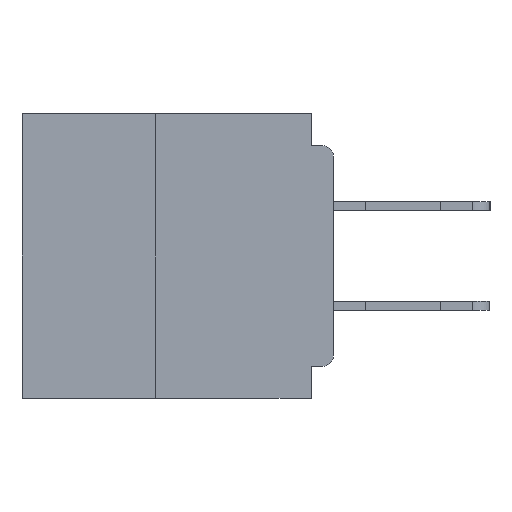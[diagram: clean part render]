
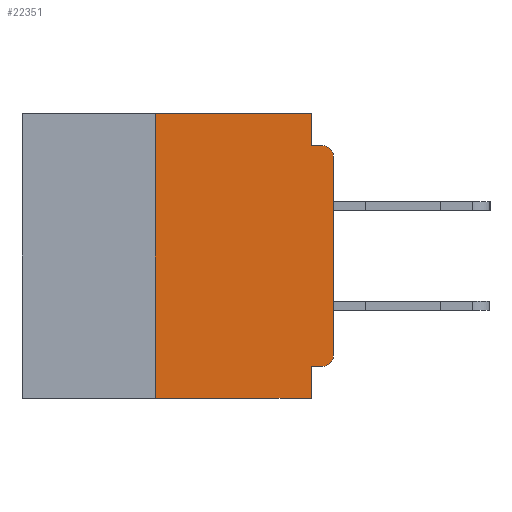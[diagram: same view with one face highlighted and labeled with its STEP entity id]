
A CAD part, left-side view. The second image highlights one B-rep face of the part: STEP entity #22351.
In plain terms, the highlighted planar face has unit normal (-1, 0, 0).
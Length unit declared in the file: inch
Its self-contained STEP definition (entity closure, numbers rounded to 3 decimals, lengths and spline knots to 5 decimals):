
#39 = VERTEX_POINT ( 'NONE', #34065 ) ;
#1166 = EDGE_CURVE ( 'NONE', #16202, #13693, #30285, .T. ) ;
#1702 = CARTESIAN_POINT ( 'NONE',  ( 0., 0., -0.045 ) ) ;
#1745 = EDGE_CURVE ( 'NONE', #2327, #4571, #15936, .T. ) ;
#2327 = VERTEX_POINT ( 'NONE', #35479 ) ;
#2402 = ORIENTED_EDGE ( 'NONE', *, *, #14206, .F. ) ;
#2523 = ORIENTED_EDGE ( 'NONE', *, *, #1745, .T. ) ;
#3564 = CARTESIAN_POINT ( 'NONE',  ( 0., 0.031, -0.4 ) ) ;
#4571 = VERTEX_POINT ( 'NONE', #23631 ) ;
#5161 = DIRECTION ( 'NONE',  ( 1., 0., 0. ) ) ;
#5773 = VERTEX_POINT ( 'NONE', #30542 ) ;
#6461 = ORIENTED_EDGE ( 'NONE', *, *, #18752, .T. ) ;
#7324 = VECTOR ( 'NONE', #26563, 39.37008 ) ;
#7698 = VECTOR ( 'NONE', #8587, 39.37008 ) ;
#8587 = DIRECTION ( 'NONE',  ( 0., 0., 1. ) ) ;
#9088 = EDGE_CURVE ( 'NONE', #33214, #16202, #17918, .T. ) ;
#9130 = LINE ( 'NONE', #1702, #14126 ) ;
#9551 = CARTESIAN_POINT ( 'NONE',  ( 0., 0.031, 0. ) ) ;
#10005 = CARTESIAN_POINT ( 'NONE',  ( 0., 0., -0.355 ) ) ;
#10224 = VECTOR ( 'NONE', #25050, 39.37008 ) ;
#10662 = DIRECTION ( 'NONE',  ( 0., -1., 0. ) ) ;
#10870 = CARTESIAN_POINT ( 'NONE',  ( 0., 0.031, 0. ) ) ;
#10946 = PLANE ( 'NONE',  #32165 ) ;
#11041 = LINE ( 'NONE', #35198, #7324 ) ;
#11042 = CARTESIAN_POINT ( 'NONE',  ( 0., 0.015, -0.34 ) ) ;
#11160 = CARTESIAN_POINT ( 'NONE',  ( 0., 0.031, -0.045 ) ) ;
#13007 = ORIENTED_EDGE ( 'NONE', *, *, #33110, .F. ) ;
#13212 = LINE ( 'NONE', #27355, #27936 ) ;
#13385 = ORIENTED_EDGE ( 'NONE', *, *, #31319, .F. ) ;
#13693 = VERTEX_POINT ( 'NONE', #11160 ) ;
#13855 = CARTESIAN_POINT ( 'NONE',  ( 0., 0.437, 0. ) ) ;
#13951 = DIRECTION ( 'NONE',  ( 0., 0., -1. ) ) ;
#14126 = VECTOR ( 'NONE', #10662, 39.37008 ) ;
#14144 = VERTEX_POINT ( 'NONE', #16159 ) ;
#14206 = EDGE_CURVE ( 'NONE', #5773, #27814, #21734, .T. ) ;
#15553 = VERTEX_POINT ( 'NONE', #28361 ) ;
#15936 = CIRCLE ( 'NONE', #16448, 0.015 ) ;
#16159 = CARTESIAN_POINT ( 'NONE',  ( 0., 0.015, -0.355 ) ) ;
#16202 = VERTEX_POINT ( 'NONE', #10870 ) ;
#16414 = CARTESIAN_POINT ( 'NONE',  ( 0., 0.031, -0.4 ) ) ;
#16448 = AXIS2_PLACEMENT_3D ( 'NONE', #22182, #21031, #35310 ) ;
#17918 = LINE ( 'NONE', #27908, #10224 ) ;
#18578 = EDGE_CURVE ( 'NONE', #13693, #4571, #9130, .T. ) ;
#18752 = EDGE_CURVE ( 'NONE', #15553, #2327, #23318, .T. ) ;
#20002 = VECTOR ( 'NONE', #33392, 39.37008 ) ;
#20537 = VECTOR ( 'NONE', #23725, 39.37008 ) ;
#21031 = DIRECTION ( 'NONE',  ( -1., 0., 0. ) ) ;
#21053 = FACE_OUTER_BOUND ( 'NONE', #37218, .T. ) ;
#21326 = AXIS2_PLACEMENT_3D ( 'NONE', #11042, #31537, #13951 ) ;
#21472 = ORIENTED_EDGE ( 'NONE', *, *, #9088, .F. ) ;
#21734 = LINE ( 'NONE', #16414, #27782 ) ;
#22182 = CARTESIAN_POINT ( 'NONE',  ( 0., 0.015, -0.06 ) ) ;
#22351 = ADVANCED_FACE ( 'NONE', ( #21053 ), #10946, .F. ) ;
#22918 = EDGE_CURVE ( 'NONE', #14144, #15553, #24308, .T. ) ;
#23318 = LINE ( 'NONE', #26151, #7698 ) ;
#23631 = CARTESIAN_POINT ( 'NONE',  ( 0., 0.015, -0.045 ) ) ;
#23725 = DIRECTION ( 'NONE',  ( 0., 0., -1. ) ) ;
#24308 = CIRCLE ( 'NONE', #21326, 0.015 ) ;
#24393 = DIRECTION ( 'NONE',  ( 0., -1., 0. ) ) ;
#24507 = ORIENTED_EDGE ( 'NONE', *, *, #22918, .T. ) ;
#24801 = ORIENTED_EDGE ( 'NONE', *, *, #18578, .F. ) ;
#25050 = DIRECTION ( 'NONE',  ( 0., -1., 0. ) ) ;
#25674 = DIRECTION ( 'NONE',  ( 0., 0., -1. ) ) ;
#25874 = ORIENTED_EDGE ( 'NONE', *, *, #26715, .T. ) ;
#26151 = CARTESIAN_POINT ( 'NONE',  ( 0., 0., 0. ) ) ;
#26563 = DIRECTION ( 'NONE',  ( 0., 0., 1. ) ) ;
#26715 = EDGE_CURVE ( 'NONE', #39, #27814, #13212, .T. ) ;
#27355 = CARTESIAN_POINT ( 'NONE',  ( 0., 0.437, -0.4 ) ) ;
#27782 = VECTOR ( 'NONE', #33985, 39.37008 ) ;
#27814 = VERTEX_POINT ( 'NONE', #3564 ) ;
#27908 = CARTESIAN_POINT ( 'NONE',  ( 0., 0.437, 0. ) ) ;
#27936 = VECTOR ( 'NONE', #24393, 39.37008 ) ;
#28361 = CARTESIAN_POINT ( 'NONE',  ( 0., 0., -0.34 ) ) ;
#30285 = LINE ( 'NONE', #9551, #20537 ) ;
#30542 = CARTESIAN_POINT ( 'NONE',  ( 0., 0.031, -0.355 ) ) ;
#31319 = EDGE_CURVE ( 'NONE', #39, #33214, #11041, .T. ) ;
#31537 = DIRECTION ( 'NONE',  ( -1., 0., 0. ) ) ;
#32165 = AXIS2_PLACEMENT_3D ( 'NONE', #13855, #5161, #25674 ) ;
#33110 = EDGE_CURVE ( 'NONE', #14144, #5773, #35593, .T. ) ;
#33214 = VERTEX_POINT ( 'NONE', #33881 ) ;
#33392 = DIRECTION ( 'NONE',  ( 0., 1., 0. ) ) ;
#33881 = CARTESIAN_POINT ( 'NONE',  ( 0., 0.25, 0. ) ) ;
#33985 = DIRECTION ( 'NONE',  ( 0., 0., -1. ) ) ;
#34065 = CARTESIAN_POINT ( 'NONE',  ( 0., 0.25, -0.4 ) ) ;
#35198 = CARTESIAN_POINT ( 'NONE',  ( 0., 0.25, -0.4 ) ) ;
#35310 = DIRECTION ( 'NONE',  ( 0., 0., -1. ) ) ;
#35479 = CARTESIAN_POINT ( 'NONE',  ( 0., 0., -0.06 ) ) ;
#35593 = LINE ( 'NONE', #10005, #20002 ) ;
#37218 = EDGE_LOOP ( 'NONE', ( #6461, #2523, #24801, #37339, #21472, #13385, #25874, #2402, #13007, #24507 ) ) ;
#37339 = ORIENTED_EDGE ( 'NONE', *, *, #1166, .F. ) ;
